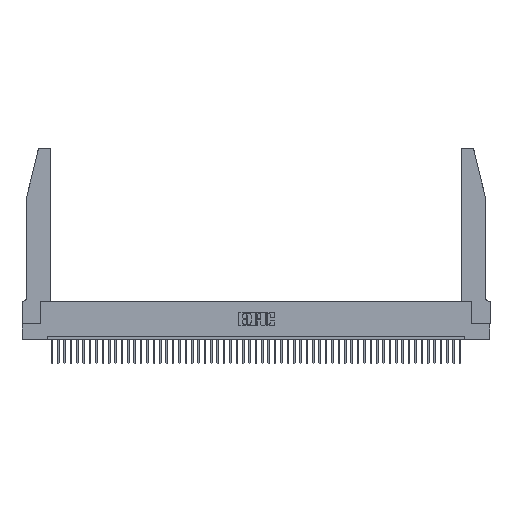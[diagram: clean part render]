
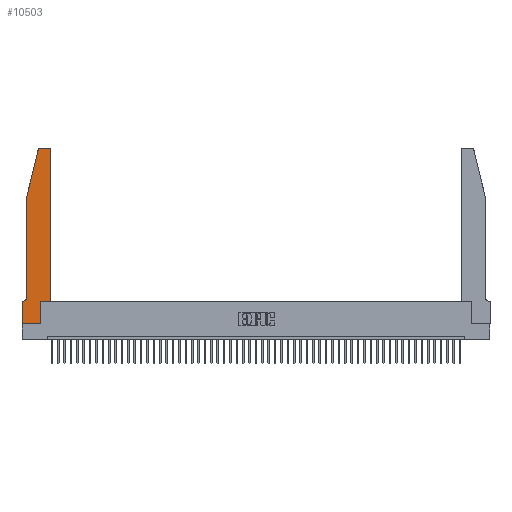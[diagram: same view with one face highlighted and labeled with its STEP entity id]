
A CAD part, top view. The second image highlights one B-rep face of the part: STEP entity #10503.
In plain terms, the highlighted planar face has unit normal (0, 0, 1).
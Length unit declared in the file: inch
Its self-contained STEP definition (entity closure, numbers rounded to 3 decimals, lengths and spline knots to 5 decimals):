
#133 = AXIS2_PLACEMENT_3D ( 'NONE', #30634, #46250, #30320 ) ;
#419 = CARTESIAN_POINT ( 'NONE',  ( 0.25487, 2.72718, 0.37 ) ) ;
#1029 = VERTEX_POINT ( 'NONE', #7320 ) ;
#1861 = VECTOR ( 'NONE', #34496, 39.37008 ) ;
#1895 = VERTEX_POINT ( 'NONE', #47127 ) ;
#1897 = EDGE_CURVE ( 'NONE', #7552, #1895, #42448, .T. ) ;
#2306 = CARTESIAN_POINT ( 'NONE',  ( 0.284, 2.72, 0.37 ) ) ;
#2314 = CARTESIAN_POINT ( 'NONE',  ( 0., 0.35, 0.37 ) ) ;
#3098 = CARTESIAN_POINT ( 'NONE',  ( 0.4505, 0.35, 0.37 ) ) ;
#3566 = CARTESIAN_POINT ( 'NONE',  ( 0.0755, 0.35, 0.37 ) ) ;
#4099 = EDGE_CURVE ( 'NONE', #46024, #1029, #5022, .T. ) ;
#5022 = CIRCLE ( 'NONE', #45069, 0.03 ) ;
#5370 = CARTESIAN_POINT ( 'NONE',  ( 0.284, 2.75, 0.37 ) ) ;
#6188 = DIRECTION ( 'NONE',  ( 0., -1., 0. ) ) ;
#6253 = CARTESIAN_POINT ( 'NONE',  ( 0.2865, 0.35, 0.37 ) ) ;
#6402 = DIRECTION ( 'NONE',  ( 0., 0., 1. ) ) ;
#6644 = VERTEX_POINT ( 'NONE', #419 ) ;
#7320 = CARTESIAN_POINT ( 'NONE',  ( 0.4205, 2.75, 0.37 ) ) ;
#7552 = VERTEX_POINT ( 'NONE', #24900 ) ;
#8174 = LINE ( 'NONE', #21966, #43562 ) ;
#10075 = VECTOR ( 'NONE', #23342, 39.37008 ) ;
#10503 = ADVANCED_FACE ( 'NONE', ( #28956 ), #18704, .T. ) ;
#10784 = ORIENTED_EDGE ( 'NONE', *, *, #13586, .T. ) ;
#10792 = CARTESIAN_POINT ( 'NONE',  ( 0.0055, 0.35, 0.37 ) ) ;
#11082 = VERTEX_POINT ( 'NONE', #2314 ) ;
#12669 = LINE ( 'NONE', #39860, #38932 ) ;
#12704 = ORIENTED_EDGE ( 'NONE', *, *, #42906, .T. ) ;
#13178 = EDGE_CURVE ( 'NONE', #15317, #11082, #37310, .T. ) ;
#13565 = DIRECTION ( 'NONE',  ( -0.239, -0.971, 0. ) ) ;
#13586 = EDGE_CURVE ( 'NONE', #30812, #15317, #25645, .T. ) ;
#13760 = LINE ( 'NONE', #42425, #25960 ) ;
#15172 = ORIENTED_EDGE ( 'NONE', *, *, #23116, .T. ) ;
#15274 = ORIENTED_EDGE ( 'NONE', *, *, #26747, .T. ) ;
#15317 = VERTEX_POINT ( 'NONE', #10792 ) ;
#15618 = CARTESIAN_POINT ( 'NONE',  ( 0.4205, 2.72, 0.37 ) ) ;
#15635 = DIRECTION ( 'NONE',  ( 0., -1., 0. ) ) ;
#15786 = ORIENTED_EDGE ( 'NONE', *, *, #42755, .T. ) ;
#16296 = LINE ( 'NONE', #21576, #45530 ) ;
#16354 = AXIS2_PLACEMENT_3D ( 'NONE', #2306, #6402, #37169 ) ;
#17494 = ORIENTED_EDGE ( 'NONE', *, *, #1897, .T. ) ;
#17827 = CARTESIAN_POINT ( 'NONE',  ( 0.0755, 2., 0.37 ) ) ;
#18020 = DIRECTION ( 'NONE',  ( 0., 1., 0. ) ) ;
#18249 = VECTOR ( 'NONE', #6188, 39.37008 ) ;
#18704 = PLANE ( 'NONE',  #133 ) ;
#18797 = ORIENTED_EDGE ( 'NONE', *, *, #13178, .T. ) ;
#21576 = CARTESIAN_POINT ( 'NONE',  ( 0.2605, 2.75, 0.37 ) ) ;
#21966 = CARTESIAN_POINT ( 'NONE',  ( 0.2865, 0.35, 0.37 ) ) ;
#22655 = EDGE_LOOP ( 'NONE', ( #30050, #15274, #12704, #42378, #10784, #18797, #15786, #17494, #24180, #32057, #15172, #49320 ) ) ;
#22962 = LINE ( 'NONE', #36802, #50331 ) ;
#23116 = EDGE_CURVE ( 'NONE', #42421, #46024, #12669, .T. ) ;
#23342 = DIRECTION ( 'NONE',  ( 1., 0., 0. ) ) ;
#23452 = EDGE_CURVE ( 'NONE', #1029, #24572, #16296, .T. ) ;
#23921 = VERTEX_POINT ( 'NONE', #45456 ) ;
#24180 = ORIENTED_EDGE ( 'NONE', *, *, #43118, .T. ) ;
#24344 = DIRECTION ( 'NONE',  ( 0., 1., 0. ) ) ;
#24572 = VERTEX_POINT ( 'NONE', #5370 ) ;
#24900 = CARTESIAN_POINT ( 'NONE',  ( 0., 0., 0.37 ) ) ;
#25624 = DIRECTION ( 'NONE',  ( 0., 0., -1. ) ) ;
#25645 = CIRCLE ( 'NONE', #37235, 0.07 ) ;
#25960 = VECTOR ( 'NONE', #15635, 39.37008 ) ;
#26747 = EDGE_CURVE ( 'NONE', #24572, #6644, #27008, .T. ) ;
#27008 = CIRCLE ( 'NONE', #16354, 0.03 ) ;
#28956 = FACE_OUTER_BOUND ( 'NONE', #22655, .T. ) ;
#29717 = CARTESIAN_POINT ( 'NONE',  ( 0.4505, 0.35, 0.37 ) ) ;
#30050 = ORIENTED_EDGE ( 'NONE', *, *, #23452, .T. ) ;
#30320 = DIRECTION ( 'NONE',  ( 1., 0., 0. ) ) ;
#30634 = CARTESIAN_POINT ( 'NONE',  ( 0., 0.35, 0.37 ) ) ;
#30812 = VERTEX_POINT ( 'NONE', #35246 ) ;
#32057 = ORIENTED_EDGE ( 'NONE', *, *, #43926, .T. ) ;
#32809 = DIRECTION ( 'NONE',  ( -1., 0., 0. ) ) ;
#33818 = CARTESIAN_POINT ( 'NONE',  ( 0.0055, 0.42, 0.37 ) ) ;
#34104 = EDGE_CURVE ( 'NONE', #23921, #30812, #47467, .T. ) ;
#34364 = DIRECTION ( 'NONE',  ( 1., 0., 0. ) ) ;
#34496 = DIRECTION ( 'NONE',  ( -1., 0., 0. ) ) ;
#35246 = CARTESIAN_POINT ( 'NONE',  ( 0.0755, 0.42, 0.37 ) ) ;
#36802 = CARTESIAN_POINT ( 'NONE',  ( 0.0755, 2., 0.37 ) ) ;
#37169 = DIRECTION ( 'NONE',  ( 1., 0., 0. ) ) ;
#37235 = AXIS2_PLACEMENT_3D ( 'NONE', #33818, #25624, #48763 ) ;
#37310 = LINE ( 'NONE', #3566, #1861 ) ;
#38060 = VECTOR ( 'NONE', #34364, 39.37008 ) ;
#38861 = CARTESIAN_POINT ( 'NONE',  ( 0., 0., 0.37 ) ) ;
#38932 = VECTOR ( 'NONE', #24344, 39.37008 ) ;
#39860 = CARTESIAN_POINT ( 'NONE',  ( 0.4505, 0.35, 0.37 ) ) ;
#40760 = VERTEX_POINT ( 'NONE', #6253 ) ;
#42378 = ORIENTED_EDGE ( 'NONE', *, *, #34104, .T. ) ;
#42421 = VERTEX_POINT ( 'NONE', #29717 ) ;
#42425 = CARTESIAN_POINT ( 'NONE',  ( 0., 0., 0.37 ) ) ;
#42448 = LINE ( 'NONE', #38861, #10075 ) ;
#42755 = EDGE_CURVE ( 'NONE', #11082, #7552, #13760, .T. ) ;
#42906 = EDGE_CURVE ( 'NONE', #6644, #23921, #22962, .T. ) ;
#43118 = EDGE_CURVE ( 'NONE', #1895, #40760, #8174, .T. ) ;
#43562 = VECTOR ( 'NONE', #18020, 39.37008 ) ;
#43926 = EDGE_CURVE ( 'NONE', #40760, #42421, #48354, .T. ) ;
#45069 = AXIS2_PLACEMENT_3D ( 'NONE', #15618, #50391, #46773 ) ;
#45456 = CARTESIAN_POINT ( 'NONE',  ( 0.0755, 2., 0.37 ) ) ;
#45530 = VECTOR ( 'NONE', #32809, 39.37008 ) ;
#45690 = CARTESIAN_POINT ( 'NONE',  ( 0.4505, 2.72, 0.37 ) ) ;
#46024 = VERTEX_POINT ( 'NONE', #45690 ) ;
#46250 = DIRECTION ( 'NONE',  ( 0., 0., 1. ) ) ;
#46773 = DIRECTION ( 'NONE',  ( 1., 0., 0. ) ) ;
#47127 = CARTESIAN_POINT ( 'NONE',  ( 0.2865, 0., 0.37 ) ) ;
#47467 = LINE ( 'NONE', #17827, #18249 ) ;
#48354 = LINE ( 'NONE', #3098, #38060 ) ;
#48763 = DIRECTION ( 'NONE',  ( -1., 0., 0. ) ) ;
#49320 = ORIENTED_EDGE ( 'NONE', *, *, #4099, .T. ) ;
#50331 = VECTOR ( 'NONE', #13565, 39.37008 ) ;
#50391 = DIRECTION ( 'NONE',  ( 0., 0., 1. ) ) ;
